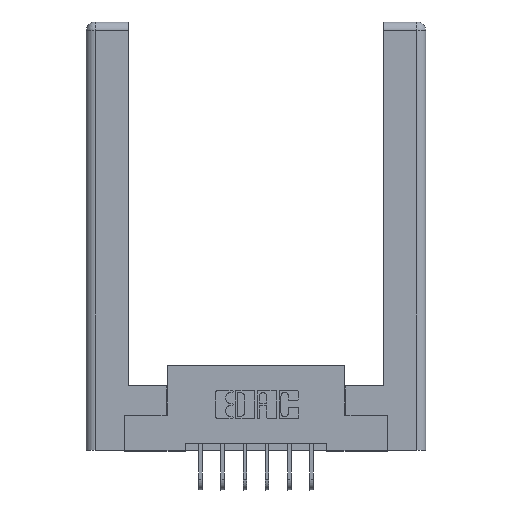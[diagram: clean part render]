
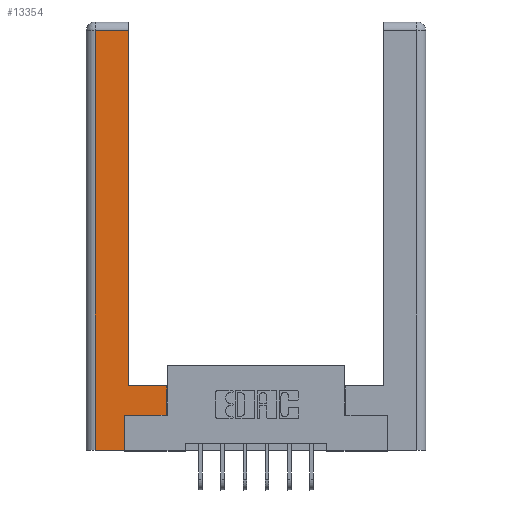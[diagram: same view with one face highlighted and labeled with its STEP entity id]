
A CAD part, top view. The second image highlights one B-rep face of the part: STEP entity #13354.
In plain terms, the highlighted planar face has unit normal (0, 0, 1).
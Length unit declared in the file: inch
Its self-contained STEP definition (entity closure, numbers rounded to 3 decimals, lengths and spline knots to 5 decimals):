
#38 = LINE ( 'NONE', #8710, #6186 ) ;
#71 = CARTESIAN_POINT ( 'NONE',  ( 0.265, 0., 0. ) ) ;
#197 = CARTESIAN_POINT ( 'NONE',  ( 0.265, 0., 0. ) ) ;
#242 = DIRECTION ( 'NONE',  ( 0., 1., 0. ) ) ;
#424 = EDGE_CURVE ( 'NONE', #13093, #9015, #5504, .T. ) ;
#550 = VERTEX_POINT ( 'NONE', #4947 ) ;
#639 = EDGE_CURVE ( 'NONE', #11093, #550, #4130, .T. ) ;
#680 = CARTESIAN_POINT ( 'NONE',  ( 0.565, 0.245, 0. ) ) ;
#1252 = DIRECTION ( 'NONE',  ( -1., 0., 0. ) ) ;
#1281 = EDGE_CURVE ( 'NONE', #550, #12775, #1797, .T. ) ;
#1309 = VERTEX_POINT ( 'NONE', #197 ) ;
#1569 = CARTESIAN_POINT ( 'NONE',  ( 0.295, 0.45, 0. ) ) ;
#1780 = EDGE_CURVE ( 'NONE', #1309, #4748, #9430, .T. ) ;
#1797 = LINE ( 'NONE', #6232, #6768 ) ;
#1853 = VERTEX_POINT ( 'NONE', #680 ) ;
#2054 = DIRECTION ( 'NONE',  ( 0., -1., 0. ) ) ;
#2341 = DIRECTION ( 'NONE',  ( 0., 0., -1. ) ) ;
#3157 = CARTESIAN_POINT ( 'NONE',  ( 0.0615, 2.94, 0. ) ) ;
#3517 = ORIENTED_EDGE ( 'NONE', *, *, #424, .T. ) ;
#3779 = LINE ( 'NONE', #71, #6463 ) ;
#4130 = LINE ( 'NONE', #3157, #12944 ) ;
#4259 = DIRECTION ( 'NONE',  ( 1., 0., 0. ) ) ;
#4748 = VERTEX_POINT ( 'NONE', #8164 ) ;
#4896 = AXIS2_PLACEMENT_3D ( 'NONE', #11768, #2341, #8646 ) ;
#4947 = CARTESIAN_POINT ( 'NONE',  ( 0.0615, 2.94, 0. ) ) ;
#5504 = LINE ( 'NONE', #7587, #11288 ) ;
#5607 = CARTESIAN_POINT ( 'NONE',  ( 0.0615, 0., 0. ) ) ;
#5682 = CARTESIAN_POINT ( 'NONE',  ( 0.295, 2.94, 0. ) ) ;
#6186 = VECTOR ( 'NONE', #242, 39.37008 ) ;
#6232 = CARTESIAN_POINT ( 'NONE',  ( 0.0615, 0., 0. ) ) ;
#6285 = EDGE_CURVE ( 'NONE', #4748, #1853, #7605, .T. ) ;
#6309 = LINE ( 'NONE', #10181, #13112 ) ;
#6310 = CARTESIAN_POINT ( 'NONE',  ( 0.565, 0.245, 0. ) ) ;
#6463 = VECTOR ( 'NONE', #12818, 39.37008 ) ;
#6546 = EDGE_CURVE ( 'NONE', #12775, #1309, #3779, .T. ) ;
#6768 = VECTOR ( 'NONE', #2054, 39.37008 ) ;
#6831 = EDGE_LOOP ( 'NONE', ( #6866, #11693, #12494, #9798, #11053, #9370, #9292, #3517 ) ) ;
#6866 = ORIENTED_EDGE ( 'NONE', *, *, #12787, .T. ) ;
#7232 = FACE_OUTER_BOUND ( 'NONE', #6831, .T. ) ;
#7587 = CARTESIAN_POINT ( 'NONE',  ( 0.295, 0.45, 0. ) ) ;
#7605 = LINE ( 'NONE', #6310, #10760 ) ;
#7975 = DIRECTION ( 'NONE',  ( 0., 1., 0. ) ) ;
#8164 = CARTESIAN_POINT ( 'NONE',  ( 0.265, 0.245, 0. ) ) ;
#8472 = DIRECTION ( 'NONE',  ( -1., 0., 0. ) ) ;
#8646 = DIRECTION ( 'NONE',  ( -1., 0., 0. ) ) ;
#8695 = PLANE ( 'NONE',  #4896 ) ;
#8710 = CARTESIAN_POINT ( 'NONE',  ( 0.295, 3., 0. ) ) ;
#9015 = VERTEX_POINT ( 'NONE', #1569 ) ;
#9065 = CARTESIAN_POINT ( 'NONE',  ( 0.265, 0.245, 0. ) ) ;
#9292 = ORIENTED_EDGE ( 'NONE', *, *, #10080, .T. ) ;
#9370 = ORIENTED_EDGE ( 'NONE', *, *, #6285, .T. ) ;
#9430 = LINE ( 'NONE', #9065, #13085 ) ;
#9798 = ORIENTED_EDGE ( 'NONE', *, *, #6546, .T. ) ;
#10080 = EDGE_CURVE ( 'NONE', #1853, #13093, #6309, .T. ) ;
#10181 = CARTESIAN_POINT ( 'NONE',  ( 0.565, 0.45, 0. ) ) ;
#10760 = VECTOR ( 'NONE', #4259, 39.37008 ) ;
#11053 = ORIENTED_EDGE ( 'NONE', *, *, #1780, .T. ) ;
#11093 = VERTEX_POINT ( 'NONE', #5682 ) ;
#11152 = DIRECTION ( 'NONE',  ( 0., 1., 0. ) ) ;
#11288 = VECTOR ( 'NONE', #1252, 39.37008 ) ;
#11693 = ORIENTED_EDGE ( 'NONE', *, *, #639, .T. ) ;
#11768 = CARTESIAN_POINT ( 'NONE',  ( 0., 0., 0. ) ) ;
#12494 = ORIENTED_EDGE ( 'NONE', *, *, #1281, .T. ) ;
#12775 = VERTEX_POINT ( 'NONE', #5607 ) ;
#12787 = EDGE_CURVE ( 'NONE', #9015, #11093, #38, .T. ) ;
#12818 = DIRECTION ( 'NONE',  ( 1., 0., 0. ) ) ;
#12944 = VECTOR ( 'NONE', #8472, 39.37008 ) ;
#13085 = VECTOR ( 'NONE', #11152, 39.37008 ) ;
#13093 = VERTEX_POINT ( 'NONE', #13583 ) ;
#13112 = VECTOR ( 'NONE', #7975, 39.37008 ) ;
#13354 = ADVANCED_FACE ( 'NONE', ( #7232 ), #8695, .F. ) ;
#13583 = CARTESIAN_POINT ( 'NONE',  ( 0.565, 0.45, 0. ) ) ;
